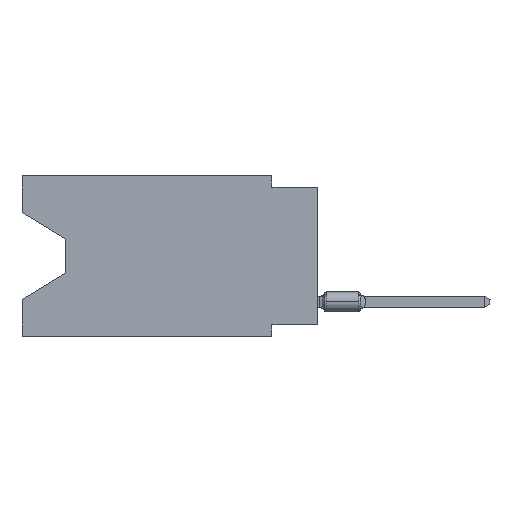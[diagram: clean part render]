
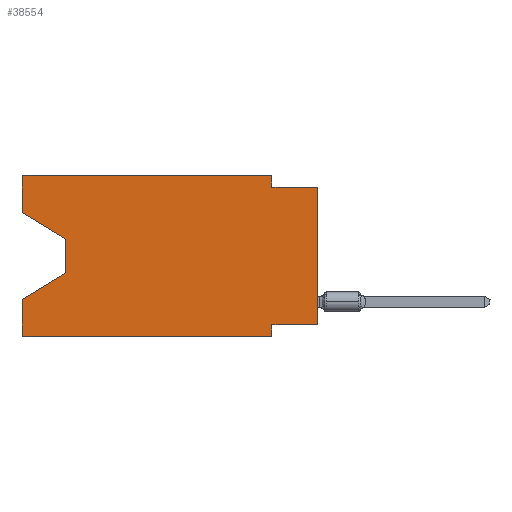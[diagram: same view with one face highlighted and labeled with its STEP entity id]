
A CAD part, left-side view. The second image highlights one B-rep face of the part: STEP entity #38554.
In plain terms, the highlighted planar face has unit normal (-1, 0, 0).
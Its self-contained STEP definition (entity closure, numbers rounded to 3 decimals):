
#1277 = CARTESIAN_POINT ( 'NONE',  ( 0., 13.97, -3.505 ) ) ;
#1296 = CARTESIAN_POINT ( 'NONE',  ( 0., 0., -8.255 ) ) ;
#2640 = CARTESIAN_POINT ( 'NONE',  ( 0., 16.383, -8.89 ) ) ;
#6848 = VERTEX_POINT ( 'NONE', #40830 ) ;
#8099 = CARTESIAN_POINT ( 'NONE',  ( 0., 16.383, 0. ) ) ;
#9199 = LINE ( 'NONE', #57258, #37586 ) ;
#14773 = CARTESIAN_POINT ( 'NONE',  ( 0., 13.97, -5.385 ) ) ;
#14878 = VECTOR ( 'NONE', #17973, 1000. ) ;
#17154 = DIRECTION ( 'NONE',  ( 0., 0.855, -0.519 ) ) ;
#17440 = ORIENTED_EDGE ( 'NONE', *, *, #72692, .T. ) ;
#17973 = DIRECTION ( 'NONE',  ( 0., 0., -1. ) ) ;
#18851 = CARTESIAN_POINT ( 'NONE',  ( 0., 13.97, -5.385 ) ) ;
#19230 = DIRECTION ( 'NONE',  ( 0., -1., 0. ) ) ;
#20501 = LINE ( 'NONE', #47406, #103633 ) ;
#22135 = VECTOR ( 'NONE', #17154, 1000. ) ;
#22561 = EDGE_CURVE ( 'NONE', #39961, #46671, #87423, .T. ) ;
#24050 = ORIENTED_EDGE ( 'NONE', *, *, #28971, .T. ) ;
#24717 = FACE_OUTER_BOUND ( 'NONE', #81568, .T. ) ;
#25662 = EDGE_CURVE ( 'NONE', #63645, #6848, #81703, .T. ) ;
#25741 = LINE ( 'NONE', #42920, #94164 ) ;
#26574 = CARTESIAN_POINT ( 'NONE',  ( 0., 2.54, -0.635 ) ) ;
#28971 = EDGE_CURVE ( 'NONE', #106221, #88360, #77877, .T. ) ;
#30206 = DIRECTION ( 'NONE',  ( 0., 0., 1. ) ) ;
#30902 = DIRECTION ( 'NONE',  ( 0., 0., -1. ) ) ;
#32858 = EDGE_CURVE ( 'NONE', #79766, #106221, #47005, .T. ) ;
#33295 = CARTESIAN_POINT ( 'NONE',  ( 0., 0., -8.255 ) ) ;
#33658 = EDGE_CURVE ( 'NONE', #57530, #39961, #91060, .T. ) ;
#36333 = ORIENTED_EDGE ( 'NONE', *, *, #36355, .F. ) ;
#36355 = EDGE_CURVE ( 'NONE', #59679, #38904, #25741, .T. ) ;
#36854 = DIRECTION ( 'NONE',  ( 0., -0.855, -0.519 ) ) ;
#37586 = VECTOR ( 'NONE', #56683, 1000. ) ;
#38554 = ADVANCED_FACE ( 'NONE', ( #24717 ), #94048, .F. ) ;
#38904 = VERTEX_POINT ( 'NONE', #104196 ) ;
#38962 = LINE ( 'NONE', #63192, #55357 ) ;
#39947 = EDGE_CURVE ( 'NONE', #101954, #6848, #69578, .T. ) ;
#39961 = VERTEX_POINT ( 'NONE', #26574 ) ;
#40188 = LINE ( 'NONE', #102592, #86557 ) ;
#40830 = CARTESIAN_POINT ( 'NONE',  ( 0., 2.54, -8.89 ) ) ;
#41691 = EDGE_CURVE ( 'NONE', #59679, #79766, #38962, .T. ) ;
#42920 = CARTESIAN_POINT ( 'NONE',  ( 0., 16.383, 0. ) ) ;
#46671 = VERTEX_POINT ( 'NONE', #86711 ) ;
#47005 = LINE ( 'NONE', #108854, #102004 ) ;
#47406 = CARTESIAN_POINT ( 'NONE',  ( 0., 16.383, 0. ) ) ;
#52481 = CARTESIAN_POINT ( 'NONE',  ( 0., 0., -0.635 ) ) ;
#53904 = DIRECTION ( 'NONE',  ( 0., 0., -1. ) ) ;
#55350 = DIRECTION ( 'NONE',  ( 0., -1., 0. ) ) ;
#55357 = VECTOR ( 'NONE', #36854, 1000. ) ;
#56683 = DIRECTION ( 'NONE',  ( 0., -1., 0. ) ) ;
#56820 = EDGE_CURVE ( 'NONE', #38904, #57530, #9199, .T. ) ;
#57258 = CARTESIAN_POINT ( 'NONE',  ( 0., 16.383, 0. ) ) ;
#57530 = VERTEX_POINT ( 'NONE', #108518 ) ;
#58361 = EDGE_CURVE ( 'NONE', #63645, #88360, #20501, .T. ) ;
#59679 = VERTEX_POINT ( 'NONE', #74470 ) ;
#60690 = DIRECTION ( 'NONE',  ( 0., 0., 1. ) ) ;
#62160 = ORIENTED_EDGE ( 'NONE', *, *, #32858, .T. ) ;
#63192 = CARTESIAN_POINT ( 'NONE',  ( 0., 16.383, -2.038 ) ) ;
#63645 = VERTEX_POINT ( 'NONE', #109371 ) ;
#65537 = VECTOR ( 'NONE', #30902, 1000. ) ;
#67621 = ORIENTED_EDGE ( 'NONE', *, *, #25662, .T. ) ;
#69578 = LINE ( 'NONE', #104493, #14878 ) ;
#70269 = CARTESIAN_POINT ( 'NONE',  ( 0., 16.383, -6.852 ) ) ;
#72195 = ORIENTED_EDGE ( 'NONE', *, *, #56820, .F. ) ;
#72692 = EDGE_CURVE ( 'NONE', #112322, #46671, #40188, .T. ) ;
#74470 = CARTESIAN_POINT ( 'NONE',  ( 0., 16.383, -2.038 ) ) ;
#76834 = DIRECTION ( 'NONE',  ( 0., 1., 0. ) ) ;
#77499 = ORIENTED_EDGE ( 'NONE', *, *, #33658, .F. ) ;
#77877 = LINE ( 'NONE', #18851, #22135 ) ;
#79766 = VERTEX_POINT ( 'NONE', #1277 ) ;
#81290 = ORIENTED_EDGE ( 'NONE', *, *, #22561, .F. ) ;
#81568 = EDGE_LOOP ( 'NONE', ( #84477, #62160, #24050, #96368, #67621, #91702, #88785, #17440, #81290, #77499, #72195, #36333 ) ) ;
#81703 = LINE ( 'NONE', #2640, #85927 ) ;
#84477 = ORIENTED_EDGE ( 'NONE', *, *, #41691, .T. ) ;
#85927 = VECTOR ( 'NONE', #55350, 1000. ) ;
#86019 = DIRECTION ( 'NONE',  ( 1., 0., 0. ) ) ;
#86557 = VECTOR ( 'NONE', #92885, 1000. ) ;
#86711 = CARTESIAN_POINT ( 'NONE',  ( 0., 0., -0.635 ) ) ;
#87423 = LINE ( 'NONE', #52481, #96471 ) ;
#88360 = VERTEX_POINT ( 'NONE', #70269 ) ;
#88785 = ORIENTED_EDGE ( 'NONE', *, *, #101736, .F. ) ;
#91060 = LINE ( 'NONE', #92764, #65537 ) ;
#91702 = ORIENTED_EDGE ( 'NONE', *, *, #39947, .F. ) ;
#92764 = CARTESIAN_POINT ( 'NONE',  ( 0., 2.54, 0. ) ) ;
#92885 = DIRECTION ( 'NONE',  ( 0., 0., 1. ) ) ;
#94048 = PLANE ( 'NONE',  #111624 ) ;
#94164 = VECTOR ( 'NONE', #60690, 1000. ) ;
#95748 = DIRECTION ( 'NONE',  ( 0., 0., -1. ) ) ;
#96270 = CARTESIAN_POINT ( 'NONE',  ( 0., 2.54, -8.255 ) ) ;
#96368 = ORIENTED_EDGE ( 'NONE', *, *, #58361, .F. ) ;
#96471 = VECTOR ( 'NONE', #19230, 1000. ) ;
#100440 = VECTOR ( 'NONE', #76834, 1000. ) ;
#101736 = EDGE_CURVE ( 'NONE', #112322, #101954, #111759, .T. ) ;
#101954 = VERTEX_POINT ( 'NONE', #96270 ) ;
#102004 = VECTOR ( 'NONE', #53904, 1000. ) ;
#102592 = CARTESIAN_POINT ( 'NONE',  ( 0., 0., 0. ) ) ;
#103633 = VECTOR ( 'NONE', #30206, 1000. ) ;
#104196 = CARTESIAN_POINT ( 'NONE',  ( 0., 16.383, 0. ) ) ;
#104493 = CARTESIAN_POINT ( 'NONE',  ( 0., 2.54, -8.89 ) ) ;
#106221 = VERTEX_POINT ( 'NONE', #14773 ) ;
#108518 = CARTESIAN_POINT ( 'NONE',  ( 0., 2.54, 0. ) ) ;
#108854 = CARTESIAN_POINT ( 'NONE',  ( 0., 13.97, -3.505 ) ) ;
#109371 = CARTESIAN_POINT ( 'NONE',  ( 0., 16.383, -8.89 ) ) ;
#111624 = AXIS2_PLACEMENT_3D ( 'NONE', #8099, #86019, #95748 ) ;
#111759 = LINE ( 'NONE', #33295, #100440 ) ;
#112322 = VERTEX_POINT ( 'NONE', #1296 ) ;
